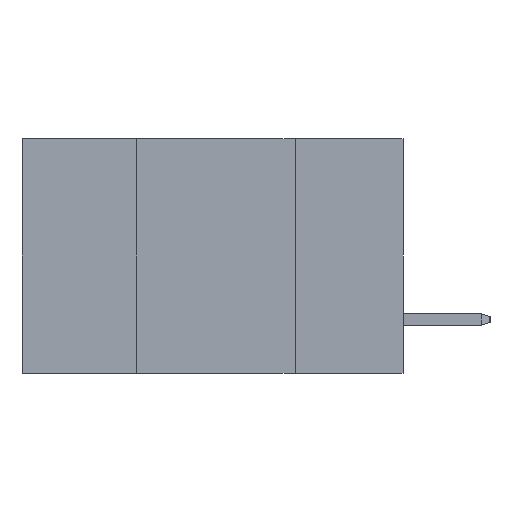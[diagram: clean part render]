
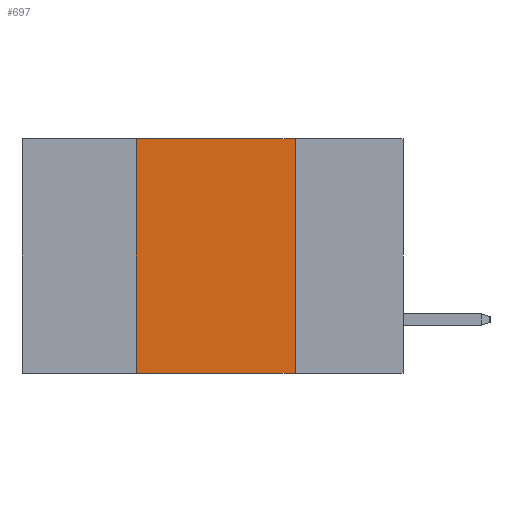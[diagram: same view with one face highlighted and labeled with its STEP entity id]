
A CAD part, left-side view. The second image highlights one B-rep face of the part: STEP entity #697.
In plain terms, the highlighted planar face has unit normal (-1, 0, 0).
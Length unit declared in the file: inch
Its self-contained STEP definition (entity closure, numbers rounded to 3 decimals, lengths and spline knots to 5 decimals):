
#498 = AXIS2_PLACEMENT_3D ( 'NONE', #11991, #12202, #9785 ) ;
#645 = ORIENTED_EDGE ( 'NONE', *, *, #9954, .T. ) ;
#697 = ADVANCED_FACE ( 'NONE', ( #11031 ), #4543, .F. ) ;
#1621 = VERTEX_POINT ( 'NONE', #9020 ) ;
#1990 = DIRECTION ( 'NONE',  ( 0., -1., 0. ) ) ;
#2560 = ORIENTED_EDGE ( 'NONE', *, *, #7894, .F. ) ;
#2717 = LINE ( 'NONE', #9286, #5803 ) ;
#2719 = DIRECTION ( 'NONE',  ( 0., 0., 1. ) ) ;
#2795 = ORIENTED_EDGE ( 'NONE', *, *, #3526, .F. ) ;
#3526 = EDGE_CURVE ( 'NONE', #11271, #1621, #3816, .T. ) ;
#3816 = LINE ( 'NONE', #7245, #13075 ) ;
#3895 = DIRECTION ( 'NONE',  ( 0., 0., -1. ) ) ;
#4543 = PLANE ( 'NONE',  #498 ) ;
#5803 = VECTOR ( 'NONE', #3895, 39.37008 ) ;
#6410 = VECTOR ( 'NONE', #1990, 39.37008 ) ;
#6818 = VERTEX_POINT ( 'NONE', #12029 ) ;
#7176 = VECTOR ( 'NONE', #10746, 39.37008 ) ;
#7245 = CARTESIAN_POINT ( 'NONE',  ( 0., 0.42, 0. ) ) ;
#7534 = VERTEX_POINT ( 'NONE', #11978 ) ;
#7894 = EDGE_CURVE ( 'NONE', #1621, #7534, #14155, .T. ) ;
#8043 = CARTESIAN_POINT ( 'NONE',  ( 0., 0.42, -0.37 ) ) ;
#9020 = CARTESIAN_POINT ( 'NONE',  ( 0., 0.42, 0. ) ) ;
#9286 = CARTESIAN_POINT ( 'NONE',  ( 0., 0.17, 0. ) ) ;
#9785 = DIRECTION ( 'NONE',  ( 0., 0., -1. ) ) ;
#9954 = EDGE_CURVE ( 'NONE', #11271, #6818, #14374, .T. ) ;
#10746 = DIRECTION ( 'NONE',  ( 0., -1., 0. ) ) ;
#11031 = FACE_OUTER_BOUND ( 'NONE', #13034, .T. ) ;
#11271 = VERTEX_POINT ( 'NONE', #8043 ) ;
#11395 = EDGE_CURVE ( 'NONE', #7534, #6818, #2717, .T. ) ;
#11731 = CARTESIAN_POINT ( 'NONE',  ( 0., 0.6, 0. ) ) ;
#11978 = CARTESIAN_POINT ( 'NONE',  ( 0., 0.17, 0. ) ) ;
#11991 = CARTESIAN_POINT ( 'NONE',  ( 0., 0.6, 0. ) ) ;
#12029 = CARTESIAN_POINT ( 'NONE',  ( 0., 0.17, -0.37 ) ) ;
#12202 = DIRECTION ( 'NONE',  ( 1., 0., 0. ) ) ;
#13034 = EDGE_LOOP ( 'NONE', ( #14422, #2560, #2795, #645 ) ) ;
#13075 = VECTOR ( 'NONE', #2719, 39.37008 ) ;
#14155 = LINE ( 'NONE', #11731, #6410 ) ;
#14226 = CARTESIAN_POINT ( 'NONE',  ( 0., 0.6, -0.37 ) ) ;
#14374 = LINE ( 'NONE', #14226, #7176 ) ;
#14422 = ORIENTED_EDGE ( 'NONE', *, *, #11395, .F. ) ;
